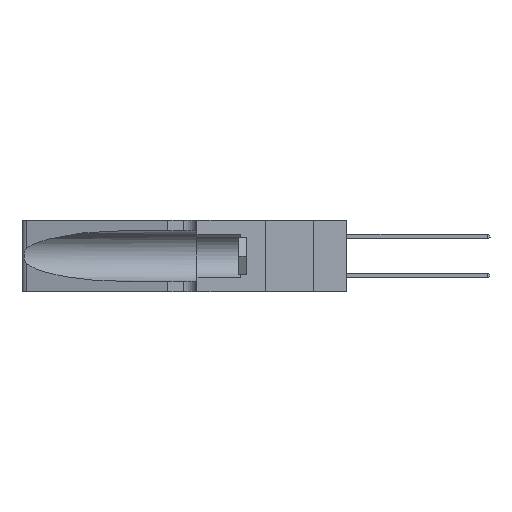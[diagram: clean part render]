
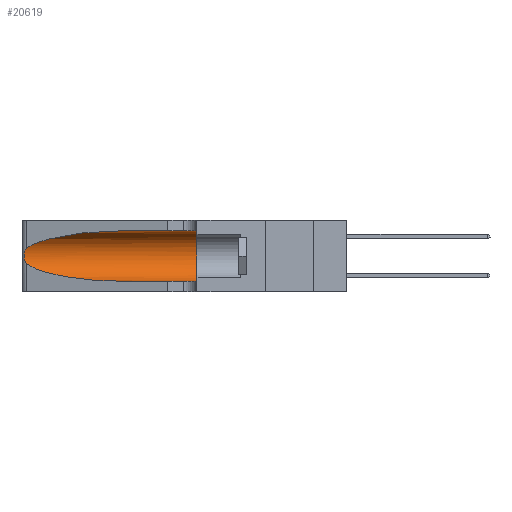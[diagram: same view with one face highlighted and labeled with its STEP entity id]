
A CAD part, left-side view. The second image highlights one B-rep face of the part: STEP entity #20619.
In plain terms, the highlighted cylindrical face has radius 3.308 mm (diameter 6.617 mm), a partial arc.
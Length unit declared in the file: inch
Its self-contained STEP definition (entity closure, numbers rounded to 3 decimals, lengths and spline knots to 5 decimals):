
#311 = LINE ( 'NONE', #24459, #982 ) ;
#618 = AXIS2_PLACEMENT_3D ( 'NONE', #1650, #26232, #22244 ) ;
#982 = VECTOR ( 'NONE', #10208, 39.37008 ) ;
#1581 = EDGE_CURVE ( 'NONE', #16083, #14203, #9056, .T. ) ;
#1650 = CARTESIAN_POINT ( 'NONE',  ( 0.1305, 1.61858, 0.185 ) ) ;
#1906 = CARTESIAN_POINT ( 'NONE',  ( 0.25487, 1.22718, 0.22369 ) ) ;
#1997 = CARTESIAN_POINT ( 'NONE',  ( 0.25854, 1.2359, 0.20912 ) ) ;
#2581 = CARTESIAN_POINT ( 'NONE',  ( 0.1305, 0.35, 0.31525 ) ) ;
#3018 = CARTESIAN_POINT ( 'NONE',  ( 0.1305, 1.61858, 0.31525 ) ) ;
#3354 = CARTESIAN_POINT ( 'NONE',  ( 0.25487, 1.22718, 0.14631 ) ) ;
#3654 = CARTESIAN_POINT ( 'NONE',  ( 0.1305, 0.35, 0.05475 ) ) ;
#4022 = CARTESIAN_POINT ( 'NONE',  ( 0.25555, 1.22994, 0.2215 ) ) ;
#4117 = CARTESIAN_POINT ( 'NONE',  ( 0.26075, 1.23896, 0.19203 ) ) ;
#4234 = CARTESIAN_POINT ( 'NONE',  ( 0.18966, 0.96281, 0.31525 ) ) ;
#5254 = CARTESIAN_POINT ( 'NONE',  ( 0.25487, 1.22718, 0.14631 ) ) ;
#5405 = VERTEX_POINT ( 'NONE', #24914 ) ;
#6198 = CARTESIAN_POINT ( 'NONE',  ( 0.26017, 1.23833, 0.17102 ) ) ;
#6303 = CARTESIAN_POINT ( 'NONE',  ( 0.25487, 1.22718, 0.22369 ) ) ;
#7340 = CARTESIAN_POINT ( 'NONE',  ( 0.1305, 0.72297, 0.05475 ) ) ;
#7678 = CARTESIAN_POINT ( 'NONE',  ( 0.1305, 0.35, 0.185 ) ) ;
#8055 = ORIENTED_EDGE ( 'NONE', *, *, #1581, .T. ) ;
#8292 = CARTESIAN_POINT ( 'NONE',  ( 0.25789, 1.23486, 0.15765 ) ) ;
#9056 =( BOUNDED_CURVE ( )  B_SPLINE_CURVE ( 3, ( #3354, #11574, #25837, #17793 ),
 .UNSPECIFIED., .F., .F. ) 
 B_SPLINE_CURVE_WITH_KNOTS ( ( 4, 4 ),
 ( 3.44316, 4.71239 ),
 .UNSPECIFIED. ) 
 CURVE ( )  GEOMETRIC_REPRESENTATION_ITEM ( )  RATIONAL_B_SPLINE_CURVE ( ( 1., 0.87, 0.87, 1. ) ) 
 REPRESENTATION_ITEM ( '' )  );
#9502 = LINE ( 'NONE', #3018, #13728 ) ;
#9635 = EDGE_CURVE ( 'NONE', #5405, #26188, #9502, .T. ) ;
#9796 = DIRECTION ( 'NONE',  ( 0., 0., 1. ) ) ;
#9894 = B_SPLINE_CURVE_WITH_KNOTS ( 'NONE', 3,
 ( #1906, #4022, #26564, #14471, #1997, #16515, #4117, #18545, #6198, #20596, #8292, #22650, #10410, #24656 ),
 .UNSPECIFIED., .F., .F.,
 ( 4, 2, 2, 2, 2, 2, 4 ),
 ( 0., 0.00027, 0.00053, 0.00107, 0.0016, 0.00187, 0.00214 ),
 .UNSPECIFIED. ) ;
#9961 = EDGE_CURVE ( 'NONE', #14203, #26469, #311, .T. ) ;
#9986 = ORIENTED_EDGE ( 'NONE', *, *, #9961, .T. ) ;
#10208 = DIRECTION ( 'NONE',  ( 0., -1., 0. ) ) ;
#10410 = CARTESIAN_POINT ( 'NONE',  ( 0.25555, 1.22993, 0.14849 ) ) ;
#10518 = CYLINDRICAL_SURFACE ( 'NONE', #618, 0.13025 ) ;
#11574 = CARTESIAN_POINT ( 'NONE',  ( 0.2373, 1.15595, 0.08982 ) ) ;
#11910 =( BOUNDED_CURVE ( )  B_SPLINE_CURVE ( 3, ( #16617, #4234, #18655, #6303 ),
 .UNSPECIFIED., .F., .F. ) 
 B_SPLINE_CURVE_WITH_KNOTS ( ( 4, 4 ),
 ( 1.5708, 2.84003 ),
 .UNSPECIFIED. ) 
 CURVE ( )  GEOMETRIC_REPRESENTATION_ITEM ( )  RATIONAL_B_SPLINE_CURVE ( ( 1., 0.87, 0.87, 1. ) ) 
 REPRESENTATION_ITEM ( '' )  );
#12029 = EDGE_CURVE ( 'NONE', #5405, #22146, #11910, .T. ) ;
#13728 = VECTOR ( 'NONE', #17451, 39.37008 ) ;
#14203 = VERTEX_POINT ( 'NONE', #7340 ) ;
#14471 = CARTESIAN_POINT ( 'NONE',  ( 0.25787, 1.23484, 0.2124 ) ) ;
#16083 = VERTEX_POINT ( 'NONE', #5254 ) ;
#16515 = CARTESIAN_POINT ( 'NONE',  ( 0.26018, 1.23835, 0.19895 ) ) ;
#16617 = CARTESIAN_POINT ( 'NONE',  ( 0.1305, 0.72297, 0.31525 ) ) ;
#17451 = DIRECTION ( 'NONE',  ( 0., -1., 0. ) ) ;
#17620 = EDGE_LOOP ( 'NONE', ( #21209, #25315, #8055, #9986, #26066, #20978 ) ) ;
#17793 = CARTESIAN_POINT ( 'NONE',  ( 0.1305, 0.72297, 0.05475 ) ) ;
#18545 = CARTESIAN_POINT ( 'NONE',  ( 0.26075, 1.23896, 0.178 ) ) ;
#18655 = CARTESIAN_POINT ( 'NONE',  ( 0.2373, 1.15595, 0.28018 ) ) ;
#19710 = EDGE_CURVE ( 'NONE', #26188, #26469, #24229, .T. ) ;
#20596 = CARTESIAN_POINT ( 'NONE',  ( 0.25856, 1.23593, 0.16098 ) ) ;
#20619 = ADVANCED_FACE ( 'NONE', ( #22021 ), #10518, .F. ) ;
#20978 = ORIENTED_EDGE ( 'NONE', *, *, #9635, .F. ) ;
#21209 = ORIENTED_EDGE ( 'NONE', *, *, #12029, .T. ) ;
#21692 = AXIS2_PLACEMENT_3D ( 'NONE', #7678, #22061, #9796 ) ;
#22021 = FACE_OUTER_BOUND ( 'NONE', #17620, .T. ) ;
#22061 = DIRECTION ( 'NONE',  ( 0., 1., 0. ) ) ;
#22146 = VERTEX_POINT ( 'NONE', #24874 ) ;
#22244 = DIRECTION ( 'NONE',  ( 0., 0., -1. ) ) ;
#22650 = CARTESIAN_POINT ( 'NONE',  ( 0.25639, 1.23186, 0.15144 ) ) ;
#24229 = CIRCLE ( 'NONE', #21692, 0.13025 ) ;
#24459 = CARTESIAN_POINT ( 'NONE',  ( 0.1305, 1.61858, 0.05475 ) ) ;
#24656 = CARTESIAN_POINT ( 'NONE',  ( 0.25487, 1.22718, 0.14631 ) ) ;
#24874 = CARTESIAN_POINT ( 'NONE',  ( 0.25487, 1.22718, 0.22369 ) ) ;
#24914 = CARTESIAN_POINT ( 'NONE',  ( 0.1305, 0.72297, 0.31525 ) ) ;
#25315 = ORIENTED_EDGE ( 'NONE', *, *, #26628, .T. ) ;
#25837 = CARTESIAN_POINT ( 'NONE',  ( 0.18966, 0.96281, 0.05475 ) ) ;
#26066 = ORIENTED_EDGE ( 'NONE', *, *, #19710, .F. ) ;
#26188 = VERTEX_POINT ( 'NONE', #2581 ) ;
#26232 = DIRECTION ( 'NONE',  ( 0., -1., 0. ) ) ;
#26469 = VERTEX_POINT ( 'NONE', #3654 ) ;
#26564 = CARTESIAN_POINT ( 'NONE',  ( 0.25639, 1.23184, 0.21858 ) ) ;
#26628 = EDGE_CURVE ( 'NONE', #22146, #16083, #9894, .T. ) ;
